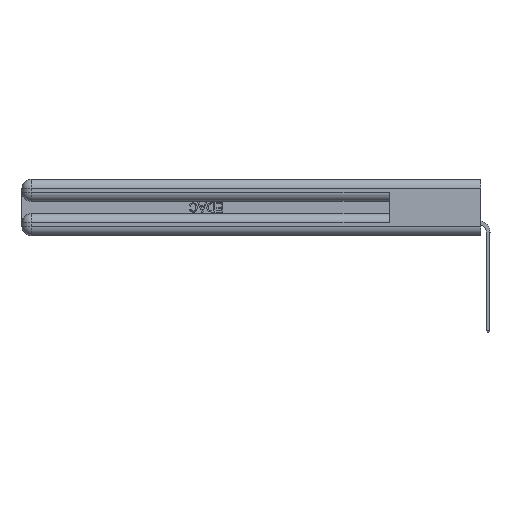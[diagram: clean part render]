
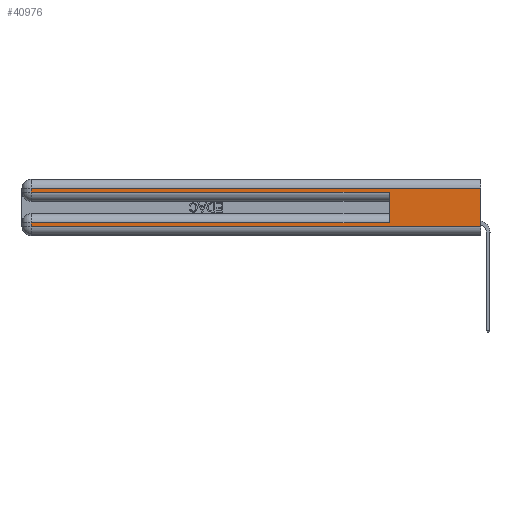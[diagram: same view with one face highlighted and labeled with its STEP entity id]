
A CAD part, left-side view. The second image highlights one B-rep face of the part: STEP entity #40976.
In plain terms, the highlighted planar face has unit normal (-1, 0, 0).
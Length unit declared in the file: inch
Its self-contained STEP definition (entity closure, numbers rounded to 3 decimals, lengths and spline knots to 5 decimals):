
#536 = FACE_OUTER_BOUND ( 'NONE', #42223, .T. ) ;
#1787 = ORIENTED_EDGE ( 'NONE', *, *, #14253, .T. ) ;
#2003 = CARTESIAN_POINT ( 'NONE',  ( 0., 2.94, 0.06 ) ) ;
#2012 = VERTEX_POINT ( 'NONE', #33092 ) ;
#5189 = VECTOR ( 'NONE', #8288, 39.37008 ) ;
#6004 = EDGE_CURVE ( 'NONE', #33616, #42179, #36621, .T. ) ;
#8288 = DIRECTION ( 'NONE',  ( 0., -1., 0. ) ) ;
#9081 = VECTOR ( 'NONE', #21793, 39.37008 ) ;
#9126 = PLANE ( 'NONE',  #22361 ) ;
#9671 = LINE ( 'NONE', #22917, #36350 ) ;
#10576 = LINE ( 'NONE', #28776, #5189 ) ;
#10995 = VECTOR ( 'NONE', #26331, 39.37008 ) ;
#11753 = EDGE_CURVE ( 'NONE', #28863, #33392, #27269, .T. ) ;
#11795 = EDGE_CURVE ( 'NONE', #27835, #2012, #34645, .T. ) ;
#14138 = ORIENTED_EDGE ( 'NONE', *, *, #24854, .T. ) ;
#14253 = EDGE_CURVE ( 'NONE', #16185, #15450, #40807, .T. ) ;
#15401 = CARTESIAN_POINT ( 'NONE',  ( 0., 2.94, 0.37 ) ) ;
#15450 = VERTEX_POINT ( 'NONE', #2003 ) ;
#16185 = VERTEX_POINT ( 'NONE', #19309 ) ;
#16291 = DIRECTION ( 'NONE',  ( 1., 0., 0. ) ) ;
#17276 = CARTESIAN_POINT ( 'NONE',  ( 0., 2.94, 0.285 ) ) ;
#18056 = CARTESIAN_POINT ( 'NONE',  ( 0., 0., 0.37 ) ) ;
#19309 = CARTESIAN_POINT ( 'NONE',  ( 0., 2.94, 0.085 ) ) ;
#20055 = LINE ( 'NONE', #36461, #10995 ) ;
#21793 = DIRECTION ( 'NONE',  ( 0., 0., -1. ) ) ;
#22222 = DIRECTION ( 'NONE',  ( 0., 0., 1. ) ) ;
#22361 = AXIS2_PLACEMENT_3D ( 'NONE', #33329, #16291, #26024 ) ;
#22739 = EDGE_CURVE ( 'NONE', #33392, #2012, #10576, .T. ) ;
#22917 = CARTESIAN_POINT ( 'NONE',  ( 0., 0., 0.06 ) ) ;
#24854 = EDGE_CURVE ( 'NONE', #15450, #42179, #9671, .T. ) ;
#25766 = VECTOR ( 'NONE', #26441, 39.37008 ) ;
#26024 = DIRECTION ( 'NONE',  ( 0., 0., -1. ) ) ;
#26072 = VECTOR ( 'NONE', #22222, 39.37008 ) ;
#26331 = DIRECTION ( 'NONE',  ( 0., 1., 0. ) ) ;
#26441 = DIRECTION ( 'NONE',  ( 0., 1., 0. ) ) ;
#26791 = DIRECTION ( 'NONE',  ( 0., -1., 0. ) ) ;
#27269 = LINE ( 'NONE', #42229, #9081 ) ;
#27835 = VERTEX_POINT ( 'NONE', #33058 ) ;
#28627 = CARTESIAN_POINT ( 'NONE',  ( 0., 0., 0.31 ) ) ;
#28776 = CARTESIAN_POINT ( 'NONE',  ( 0., 0., 0.285 ) ) ;
#28863 = VERTEX_POINT ( 'NONE', #40100 ) ;
#29759 = CARTESIAN_POINT ( 'NONE',  ( 0., 0., 0.31 ) ) ;
#30125 = EDGE_CURVE ( 'NONE', #33616, #28863, #32720, .T. ) ;
#32720 = LINE ( 'NONE', #29759, #25766 ) ;
#33058 = CARTESIAN_POINT ( 'NONE',  ( 0., 0.6, 0.085 ) ) ;
#33092 = CARTESIAN_POINT ( 'NONE',  ( 0., 0.6, 0.285 ) ) ;
#33329 = CARTESIAN_POINT ( 'NONE',  ( 0., 0., 0.37 ) ) ;
#33392 = VERTEX_POINT ( 'NONE', #17276 ) ;
#33616 = VERTEX_POINT ( 'NONE', #28627 ) ;
#34645 = LINE ( 'NONE', #35957, #26072 ) ;
#34914 = ORIENTED_EDGE ( 'NONE', *, *, #30125, .T. ) ;
#35228 = ORIENTED_EDGE ( 'NONE', *, *, #38511, .T. ) ;
#35731 = DIRECTION ( 'NONE',  ( 0., 0., -1. ) ) ;
#35957 = CARTESIAN_POINT ( 'NONE',  ( 0., 0.6, 0.145 ) ) ;
#36350 = VECTOR ( 'NONE', #26791, 39.37008 ) ;
#36461 = CARTESIAN_POINT ( 'NONE',  ( 0., 0., 0.085 ) ) ;
#36509 = VECTOR ( 'NONE', #35731, 39.37008 ) ;
#36621 = LINE ( 'NONE', #18056, #41984 ) ;
#38271 = ORIENTED_EDGE ( 'NONE', *, *, #6004, .F. ) ;
#38461 = ORIENTED_EDGE ( 'NONE', *, *, #11795, .F. ) ;
#38511 = EDGE_CURVE ( 'NONE', #27835, #16185, #20055, .T. ) ;
#38641 = DIRECTION ( 'NONE',  ( 0., 0., -1. ) ) ;
#40100 = CARTESIAN_POINT ( 'NONE',  ( 0., 2.94, 0.31 ) ) ;
#40807 = LINE ( 'NONE', #15401, #36509 ) ;
#40976 = ADVANCED_FACE ( 'NONE', ( #536 ), #9126, .F. ) ;
#41624 = ORIENTED_EDGE ( 'NONE', *, *, #22739, .T. ) ;
#41984 = VECTOR ( 'NONE', #38641, 39.37008 ) ;
#42167 = ORIENTED_EDGE ( 'NONE', *, *, #11753, .T. ) ;
#42179 = VERTEX_POINT ( 'NONE', #43373 ) ;
#42223 = EDGE_LOOP ( 'NONE', ( #38271, #34914, #42167, #41624, #38461, #35228, #1787, #14138 ) ) ;
#42229 = CARTESIAN_POINT ( 'NONE',  ( 0., 2.94, 0.37 ) ) ;
#43373 = CARTESIAN_POINT ( 'NONE',  ( 0., 0., 0.06 ) ) ;
